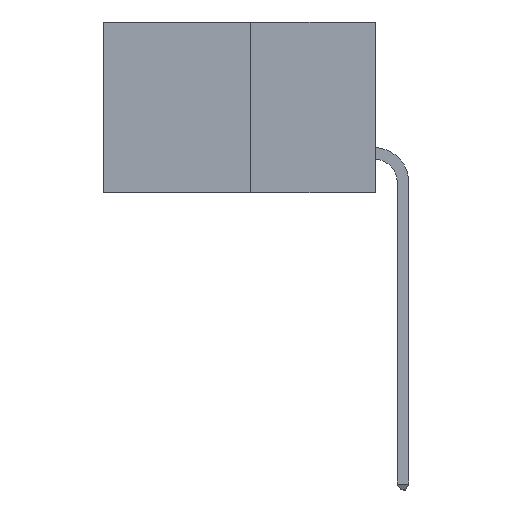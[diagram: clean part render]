
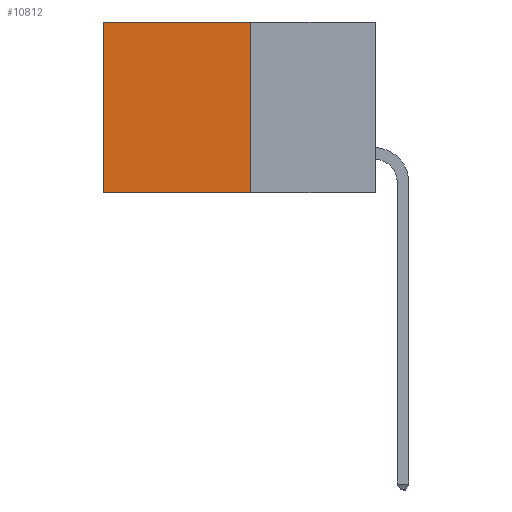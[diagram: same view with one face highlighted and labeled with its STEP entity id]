
A CAD part, left-side view. The second image highlights one B-rep face of the part: STEP entity #10812.
In plain terms, the highlighted planar face has unit normal (-1, 0, 0).
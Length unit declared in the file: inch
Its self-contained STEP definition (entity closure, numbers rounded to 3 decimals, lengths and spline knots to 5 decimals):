
#380 = CARTESIAN_POINT ( 'NONE',  ( 0.277, 0.27, -0.37 ) ) ;
#457 = VECTOR ( 'NONE', #13704, 39.37008 ) ;
#679 = ORIENTED_EDGE ( 'NONE', *, *, #5565, .F. ) ;
#1441 = VERTEX_POINT ( 'NONE', #4412 ) ;
#1726 = VERTEX_POINT ( 'NONE', #17071 ) ;
#1869 = DIRECTION ( 'NONE',  ( 1., 0., 0. ) ) ;
#2770 = LINE ( 'NONE', #9677, #16240 ) ;
#3144 = DIRECTION ( 'NONE',  ( 0., 1., 0. ) ) ;
#3172 = CARTESIAN_POINT ( 'NONE',  ( 0.277, 0.27, -0.37 ) ) ;
#4412 = CARTESIAN_POINT ( 'NONE',  ( 0.277, 0.59, -0.37 ) ) ;
#4652 = CARTESIAN_POINT ( 'NONE',  ( 0.277, 0.27, 0. ) ) ;
#5420 = VERTEX_POINT ( 'NONE', #9173 ) ;
#5565 = EDGE_CURVE ( 'NONE', #16717, #1441, #10726, .T. ) ;
#8158 = LINE ( 'NONE', #4652, #11751 ) ;
#8322 = DIRECTION ( 'NONE',  ( 0., 0., -1. ) ) ;
#8613 = ORIENTED_EDGE ( 'NONE', *, *, #11253, .F. ) ;
#8676 = CARTESIAN_POINT ( 'NONE',  ( 0.277, 0.27, -0.37 ) ) ;
#8972 = ORIENTED_EDGE ( 'NONE', *, *, #14891, .T. ) ;
#9173 = CARTESIAN_POINT ( 'NONE',  ( 0.277, 0.59, 0. ) ) ;
#9332 = ORIENTED_EDGE ( 'NONE', *, *, #15385, .T. ) ;
#9677 = CARTESIAN_POINT ( 'NONE',  ( 0.277, 0.27, -0.37 ) ) ;
#10002 = PLANE ( 'NONE',  #12451 ) ;
#10726 = LINE ( 'NONE', #380, #13834 ) ;
#10812 = ADVANCED_FACE ( 'NONE', ( #15857 ), #10002, .F. ) ;
#10886 = LINE ( 'NONE', #12366, #457 ) ;
#11253 = EDGE_CURVE ( 'NONE', #1726, #16717, #2770, .T. ) ;
#11345 = DIRECTION ( 'NONE',  ( 0., 0., -1. ) ) ;
#11751 = VECTOR ( 'NONE', #14067, 39.37008 ) ;
#12366 = CARTESIAN_POINT ( 'NONE',  ( 0.277, 0.59, -0.37 ) ) ;
#12451 = AXIS2_PLACEMENT_3D ( 'NONE', #3172, #1869, #11345 ) ;
#13704 = DIRECTION ( 'NONE',  ( 0., 0., -1. ) ) ;
#13834 = VECTOR ( 'NONE', #3144, 39.37008 ) ;
#14067 = DIRECTION ( 'NONE',  ( 0., 1., 0. ) ) ;
#14891 = EDGE_CURVE ( 'NONE', #1726, #5420, #8158, .T. ) ;
#15245 = EDGE_LOOP ( 'NONE', ( #9332, #679, #8613, #8972 ) ) ;
#15385 = EDGE_CURVE ( 'NONE', #5420, #1441, #10886, .T. ) ;
#15857 = FACE_OUTER_BOUND ( 'NONE', #15245, .T. ) ;
#16240 = VECTOR ( 'NONE', #8322, 39.37008 ) ;
#16717 = VERTEX_POINT ( 'NONE', #8676 ) ;
#17071 = CARTESIAN_POINT ( 'NONE',  ( 0.277, 0.27, 0. ) ) ;
